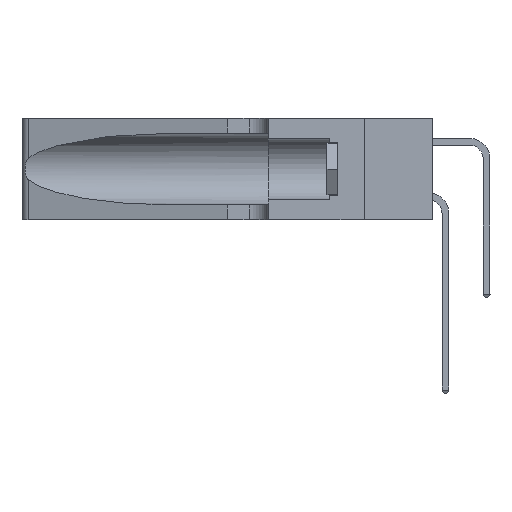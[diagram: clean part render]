
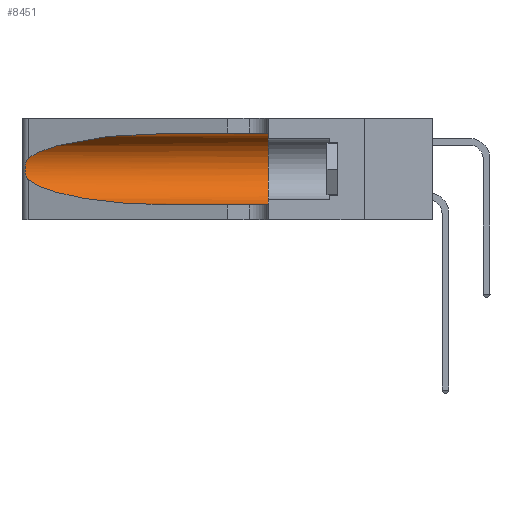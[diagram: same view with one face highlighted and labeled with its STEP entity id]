
A CAD part, left-side view. The second image highlights one B-rep face of the part: STEP entity #8451.
In plain terms, the highlighted cylindrical face has radius 3.308 mm (diameter 6.617 mm), a partial arc.
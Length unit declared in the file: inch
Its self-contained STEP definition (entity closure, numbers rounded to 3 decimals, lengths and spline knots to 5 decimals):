
#291 = DIRECTION ( 'NONE',  ( 0., 1., 0. ) ) ;
#561 = EDGE_CURVE ( 'NONE', #14208, #14426, #18365, .T. ) ;
#1559 = EDGE_CURVE ( 'NONE', #19418, #14191, #9053, .T. ) ;
#1781 = EDGE_LOOP ( 'NONE', ( #15394, #6429, #21609, #14653, #3952, #3333 ) ) ;
#1907 = AXIS2_PLACEMENT_3D ( 'NONE', #11627, #291, #13471 ) ;
#2149 = CARTESIAN_POINT ( 'NONE',  ( 0.1305, 1.61858, 0.185 ) ) ;
#2650 = CARTESIAN_POINT ( 'NONE',  ( 0.1305, 0.72297, 0.31525 ) ) ;
#3333 = ORIENTED_EDGE ( 'NONE', *, *, #561, .F. ) ;
#3952 = ORIENTED_EDGE ( 'NONE', *, *, #12373, .F. ) ;
#4430 = CARTESIAN_POINT ( 'NONE',  ( 0.1305, 1.61858, 0.31525 ) ) ;
#4692 = VERTEX_POINT ( 'NONE', #18591 ) ;
#4972 = CARTESIAN_POINT ( 'NONE',  ( 0.25487, 1.22718, 0.14631 ) ) ;
#5298 = AXIS2_PLACEMENT_3D ( 'NONE', #2149, #18696, #7845 ) ;
#6429 = ORIENTED_EDGE ( 'NONE', *, *, #1559, .T. ) ;
#6446 = CARTESIAN_POINT ( 'NONE',  ( 0.25487, 1.22718, 0.22369 ) ) ;
#6628 = EDGE_CURVE ( 'NONE', #14208, #19418, #8012, .T. ) ;
#6635 = VECTOR ( 'NONE', #7757, 39.37008 ) ;
#6675 =( BOUNDED_CURVE ( )  B_SPLINE_CURVE ( 3, ( #4972, #17799, #10590, #23125 ),
 .UNSPECIFIED., .F., .F. ) 
 B_SPLINE_CURVE_WITH_KNOTS ( ( 4, 4 ),
 ( 3.44316, 4.71239 ),
 .UNSPECIFIED. ) 
 CURVE ( )  GEOMETRIC_REPRESENTATION_ITEM ( )  RATIONAL_B_SPLINE_CURVE ( ( 1., 0.87, 0.87, 1. ) ) 
 REPRESENTATION_ITEM ( '' )  );
#7151 = CARTESIAN_POINT ( 'NONE',  ( 0.25487, 1.22718, 0.14631 ) ) ;
#7234 = CARTESIAN_POINT ( 'NONE',  ( 0.25555, 1.22993, 0.14849 ) ) ;
#7290 = CARTESIAN_POINT ( 'NONE',  ( 0.25639, 1.23186, 0.15144 ) ) ;
#7404 = CARTESIAN_POINT ( 'NONE',  ( 0.25789, 1.23486, 0.15765 ) ) ;
#7433 = CARTESIAN_POINT ( 'NONE',  ( 0.25856, 1.23593, 0.16098 ) ) ;
#7481 = CARTESIAN_POINT ( 'NONE',  ( 0.26017, 1.23833, 0.17102 ) ) ;
#7634 = CARTESIAN_POINT ( 'NONE',  ( 0.26075, 1.23896, 0.178 ) ) ;
#7712 = VERTEX_POINT ( 'NONE', #22153 ) ;
#7757 = DIRECTION ( 'NONE',  ( 0., -1., 0. ) ) ;
#7845 = DIRECTION ( 'NONE',  ( 0., 0., -1. ) ) ;
#8012 =( BOUNDED_CURVE ( )  B_SPLINE_CURVE ( 3, ( #2650, #13816, #17399, #6446 ),
 .UNSPECIFIED., .F., .T. ) 
 B_SPLINE_CURVE_WITH_KNOTS ( ( 4, 4 ),
 ( 1.5708, 2.84003 ),
 .UNSPECIFIED. ) 
 CURVE ( )  GEOMETRIC_REPRESENTATION_ITEM ( )  RATIONAL_B_SPLINE_CURVE ( ( 1., 0.87, 0.87, 1. ) ) 
 REPRESENTATION_ITEM ( '' )  );
#8451 = ADVANCED_FACE ( 'NONE', ( #19167 ), #18625, .F. ) ;
#8788 = CARTESIAN_POINT ( 'NONE',  ( 0.25639, 1.23184, 0.21858 ) ) ;
#8871 = CARTESIAN_POINT ( 'NONE',  ( 0.25854, 1.2359, 0.20912 ) ) ;
#9053 = B_SPLINE_CURVE_WITH_KNOTS ( 'NONE', 3,
 ( #9444, #9265, #8788, #9316, #8871, #9521, #9126, #7634, #7481, #7433, #7404, #7290, #7234, #7151 ),
 .UNSPECIFIED., .F., .F.,
 ( 4, 2, 2, 2, 2, 2, 4 ),
 ( 0., 0.00027, 0.00053, 0.00107, 0.0016, 0.00187, 0.00214 ),
 .UNSPECIFIED. ) ;
#9126 = CARTESIAN_POINT ( 'NONE',  ( 0.26075, 1.23896, 0.19203 ) ) ;
#9265 = CARTESIAN_POINT ( 'NONE',  ( 0.25555, 1.22994, 0.2215 ) ) ;
#9316 = CARTESIAN_POINT ( 'NONE',  ( 0.25787, 1.23484, 0.2124 ) ) ;
#9444 = CARTESIAN_POINT ( 'NONE',  ( 0.25487, 1.22718, 0.22369 ) ) ;
#9521 = CARTESIAN_POINT ( 'NONE',  ( 0.26018, 1.23835, 0.19895 ) ) ;
#10590 = CARTESIAN_POINT ( 'NONE',  ( 0.18966, 0.96281, 0.05475 ) ) ;
#11627 = CARTESIAN_POINT ( 'NONE',  ( 0.1305, 0.35, 0.185 ) ) ;
#12373 = EDGE_CURVE ( 'NONE', #14426, #7712, #23722, .T. ) ;
#13471 = DIRECTION ( 'NONE',  ( 0., 0., 1. ) ) ;
#13580 = CARTESIAN_POINT ( 'NONE',  ( 0.1305, 0.35, 0.31525 ) ) ;
#13623 = VECTOR ( 'NONE', #22688, 39.37008 ) ;
#13816 = CARTESIAN_POINT ( 'NONE',  ( 0.18966, 0.96281, 0.31525 ) ) ;
#13958 = EDGE_CURVE ( 'NONE', #14191, #4692, #6675, .T. ) ;
#14191 = VERTEX_POINT ( 'NONE', #22261 ) ;
#14208 = VERTEX_POINT ( 'NONE', #17002 ) ;
#14426 = VERTEX_POINT ( 'NONE', #13580 ) ;
#14653 = ORIENTED_EDGE ( 'NONE', *, *, #19412, .T. ) ;
#15394 = ORIENTED_EDGE ( 'NONE', *, *, #6628, .T. ) ;
#16843 = CARTESIAN_POINT ( 'NONE',  ( 0.25487, 1.22718, 0.22369 ) ) ;
#17002 = CARTESIAN_POINT ( 'NONE',  ( 0.1305, 0.72297, 0.31525 ) ) ;
#17399 = CARTESIAN_POINT ( 'NONE',  ( 0.2373, 1.15595, 0.28018 ) ) ;
#17799 = CARTESIAN_POINT ( 'NONE',  ( 0.2373, 1.15595, 0.08982 ) ) ;
#18365 = LINE ( 'NONE', #4430, #13623 ) ;
#18591 = CARTESIAN_POINT ( 'NONE',  ( 0.1305, 0.72297, 0.05475 ) ) ;
#18616 = CARTESIAN_POINT ( 'NONE',  ( 0.1305, 1.61858, 0.05475 ) ) ;
#18625 = CYLINDRICAL_SURFACE ( 'NONE', #5298, 0.13025 ) ;
#18696 = DIRECTION ( 'NONE',  ( 0., -1., 0. ) ) ;
#19167 = FACE_OUTER_BOUND ( 'NONE', #1781, .T. ) ;
#19412 = EDGE_CURVE ( 'NONE', #4692, #7712, #20517, .T. ) ;
#19418 = VERTEX_POINT ( 'NONE', #16843 ) ;
#20517 = LINE ( 'NONE', #18616, #6635 ) ;
#21609 = ORIENTED_EDGE ( 'NONE', *, *, #13958, .T. ) ;
#22153 = CARTESIAN_POINT ( 'NONE',  ( 0.1305, 0.35, 0.05475 ) ) ;
#22261 = CARTESIAN_POINT ( 'NONE',  ( 0.25487, 1.22718, 0.14631 ) ) ;
#22688 = DIRECTION ( 'NONE',  ( 0., -1., 0. ) ) ;
#23125 = CARTESIAN_POINT ( 'NONE',  ( 0.1305, 0.72297, 0.05475 ) ) ;
#23722 = CIRCLE ( 'NONE', #1907, 0.13025 ) ;
